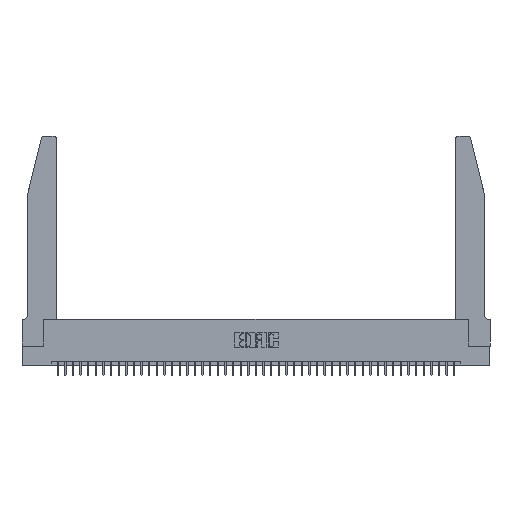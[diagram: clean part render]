
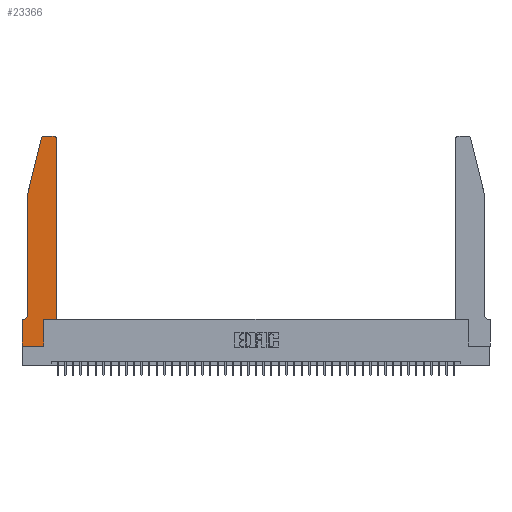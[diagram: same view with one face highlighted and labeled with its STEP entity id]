
A CAD part, top view. The second image highlights one B-rep face of the part: STEP entity #23366.
In plain terms, the highlighted planar face has unit normal (0, 0, 1).
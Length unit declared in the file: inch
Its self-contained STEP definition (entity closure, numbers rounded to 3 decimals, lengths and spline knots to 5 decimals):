
#129 = DIRECTION ( 'NONE',  ( 0., 1., 0. ) ) ;
#904 = ORIENTED_EDGE ( 'NONE', *, *, #10181, .T. ) ;
#1175 = ORIENTED_EDGE ( 'NONE', *, *, #5664, .T. ) ;
#2335 = ORIENTED_EDGE ( 'NONE', *, *, #37423, .T. ) ;
#2503 = LINE ( 'NONE', #16381, #4380 ) ;
#2833 = DIRECTION ( 'NONE',  ( 1., 0., 0. ) ) ;
#3276 = AXIS2_PLACEMENT_3D ( 'NONE', #43817, #40425, #36788 ) ;
#3529 = AXIS2_PLACEMENT_3D ( 'NONE', #12852, #26526, #24025 ) ;
#3809 = CARTESIAN_POINT ( 'NONE',  ( 0., 0.35, 0.37 ) ) ;
#4298 = VERTEX_POINT ( 'NONE', #38817 ) ;
#4380 = VECTOR ( 'NONE', #23457, 39.37008 ) ;
#5245 = LINE ( 'NONE', #39628, #39084 ) ;
#5451 = ORIENTED_EDGE ( 'NONE', *, *, #40570, .T. ) ;
#5664 = EDGE_CURVE ( 'NONE', #42920, #33251, #24505, .T. ) ;
#5913 = DIRECTION ( 'NONE',  ( 0., 1., 0. ) ) ;
#5973 = LINE ( 'NONE', #8941, #38480 ) ;
#6013 = LINE ( 'NONE', #20572, #33003 ) ;
#7016 = EDGE_CURVE ( 'NONE', #10282, #26525, #2503, .T. ) ;
#7324 = CARTESIAN_POINT ( 'NONE',  ( 0.2865, 0.35, 0.37 ) ) ;
#7619 = EDGE_CURVE ( 'NONE', #35873, #39722, #5973, .T. ) ;
#7812 = EDGE_LOOP ( 'NONE', ( #14231, #904, #12488, #36674, #24455, #23927, #14611, #23349, #5451, #9015, #1175, #2335 ) ) ;
#8283 = VECTOR ( 'NONE', #10726, 39.37008 ) ;
#8941 = CARTESIAN_POINT ( 'NONE',  ( 0.2605, 2.75, 0.37 ) ) ;
#9015 = ORIENTED_EDGE ( 'NONE', *, *, #35864, .T. ) ;
#9050 = CARTESIAN_POINT ( 'NONE',  ( 0.0755, 0.35, 0.37 ) ) ;
#9737 = CARTESIAN_POINT ( 'NONE',  ( 0.4205, 2.75, 0.37 ) ) ;
#9838 = DIRECTION ( 'NONE',  ( 0., -1., 0. ) ) ;
#10181 = EDGE_CURVE ( 'NONE', #39722, #10282, #28650, .T. ) ;
#10210 = DIRECTION ( 'NONE',  ( 1., 0., 0. ) ) ;
#10282 = VERTEX_POINT ( 'NONE', #36756 ) ;
#10448 = EDGE_CURVE ( 'NONE', #4298, #36068, #6013, .T. ) ;
#10726 = DIRECTION ( 'NONE',  ( 0., -1., 0. ) ) ;
#11253 = CIRCLE ( 'NONE', #3276, 0.03 ) ;
#11283 = CARTESIAN_POINT ( 'NONE',  ( 0.2865, 0., 0.37 ) ) ;
#12488 = ORIENTED_EDGE ( 'NONE', *, *, #7016, .T. ) ;
#12852 = CARTESIAN_POINT ( 'NONE',  ( 0.0055, 0.42, 0.37 ) ) ;
#12903 = DIRECTION ( 'NONE',  ( -1., 0., 0. ) ) ;
#14231 = ORIENTED_EDGE ( 'NONE', *, *, #7619, .T. ) ;
#14611 = ORIENTED_EDGE ( 'NONE', *, *, #40240, .T. ) ;
#15180 = CARTESIAN_POINT ( 'NONE',  ( 0.0755, 0.42, 0.37 ) ) ;
#15213 = VECTOR ( 'NONE', #129, 39.37008 ) ;
#16381 = CARTESIAN_POINT ( 'NONE',  ( 0.0755, 2., 0.37 ) ) ;
#16571 = CARTESIAN_POINT ( 'NONE',  ( 0.0055, 0.35, 0.37 ) ) ;
#16766 = VERTEX_POINT ( 'NONE', #3809 ) ;
#16777 = CARTESIAN_POINT ( 'NONE',  ( 0., 0.35, 0.37 ) ) ;
#17036 = DIRECTION ( 'NONE',  ( 0., 0., 1. ) ) ;
#20313 = LINE ( 'NONE', #41241, #44854 ) ;
#20572 = CARTESIAN_POINT ( 'NONE',  ( 0., 0., 0.37 ) ) ;
#20675 = CARTESIAN_POINT ( 'NONE',  ( 0.284, 2.72, 0.37 ) ) ;
#21361 = AXIS2_PLACEMENT_3D ( 'NONE', #20675, #17036, #10210 ) ;
#21593 = CIRCLE ( 'NONE', #3529, 0.07 ) ;
#22819 = VECTOR ( 'NONE', #26368, 39.37008 ) ;
#23219 = CARTESIAN_POINT ( 'NONE',  ( 0.4505, 0.35, 0.37 ) ) ;
#23349 = ORIENTED_EDGE ( 'NONE', *, *, #10448, .T. ) ;
#23366 = ADVANCED_FACE ( 'NONE', ( #23626 ), #34074, .T. ) ;
#23457 = DIRECTION ( 'NONE',  ( -0.239, -0.971, 0. ) ) ;
#23626 = FACE_OUTER_BOUND ( 'NONE', #7812, .T. ) ;
#23636 = LINE ( 'NONE', #37508, #22819 ) ;
#23927 = ORIENTED_EDGE ( 'NONE', *, *, #34401, .T. ) ;
#24025 = DIRECTION ( 'NONE',  ( -1., 0., 0. ) ) ;
#24455 = ORIENTED_EDGE ( 'NONE', *, *, #41676, .T. ) ;
#24505 = LINE ( 'NONE', #31543, #15213 ) ;
#26357 = AXIS2_PLACEMENT_3D ( 'NONE', #16777, #29782, #33623 ) ;
#26368 = DIRECTION ( 'NONE',  ( 1., 0., 0. ) ) ;
#26525 = VERTEX_POINT ( 'NONE', #44440 ) ;
#26526 = DIRECTION ( 'NONE',  ( 0., 0., -1. ) ) ;
#28650 = CIRCLE ( 'NONE', #21361, 0.03 ) ;
#29678 = DIRECTION ( 'NONE',  ( -1., 0., 0. ) ) ;
#29782 = DIRECTION ( 'NONE',  ( 0., 0., 1. ) ) ;
#31009 = VERTEX_POINT ( 'NONE', #16571 ) ;
#31230 = CARTESIAN_POINT ( 'NONE',  ( 0.0755, 2., 0.37 ) ) ;
#31543 = CARTESIAN_POINT ( 'NONE',  ( 0.4505, 0.35, 0.37 ) ) ;
#32774 = VERTEX_POINT ( 'NONE', #15180 ) ;
#33003 = VECTOR ( 'NONE', #2833, 39.37008 ) ;
#33251 = VERTEX_POINT ( 'NONE', #43557 ) ;
#33623 = DIRECTION ( 'NONE',  ( 1., 0., 0. ) ) ;
#34074 = PLANE ( 'NONE',  #26357 ) ;
#34401 = EDGE_CURVE ( 'NONE', #31009, #16766, #40232, .T. ) ;
#34977 = VERTEX_POINT ( 'NONE', #7324 ) ;
#35085 = EDGE_CURVE ( 'NONE', #26525, #32774, #41904, .T. ) ;
#35864 = EDGE_CURVE ( 'NONE', #34977, #42920, #23636, .T. ) ;
#35873 = VERTEX_POINT ( 'NONE', #9737 ) ;
#36068 = VERTEX_POINT ( 'NONE', #11283 ) ;
#36674 = ORIENTED_EDGE ( 'NONE', *, *, #35085, .T. ) ;
#36756 = CARTESIAN_POINT ( 'NONE',  ( 0.25487, 2.72718, 0.37 ) ) ;
#36788 = DIRECTION ( 'NONE',  ( 1., 0., 0. ) ) ;
#37423 = EDGE_CURVE ( 'NONE', #33251, #35873, #11253, .T. ) ;
#37508 = CARTESIAN_POINT ( 'NONE',  ( 0.4505, 0.35, 0.37 ) ) ;
#38480 = VECTOR ( 'NONE', #29678, 39.37008 ) ;
#38817 = CARTESIAN_POINT ( 'NONE',  ( 0., 0., 0.37 ) ) ;
#39084 = VECTOR ( 'NONE', #5913, 39.37008 ) ;
#39628 = CARTESIAN_POINT ( 'NONE',  ( 0.2865, 0.35, 0.37 ) ) ;
#39722 = VERTEX_POINT ( 'NONE', #42737 ) ;
#40232 = LINE ( 'NONE', #9050, #41712 ) ;
#40240 = EDGE_CURVE ( 'NONE', #16766, #4298, #20313, .T. ) ;
#40425 = DIRECTION ( 'NONE',  ( 0., 0., 1. ) ) ;
#40570 = EDGE_CURVE ( 'NONE', #36068, #34977, #5245, .T. ) ;
#41241 = CARTESIAN_POINT ( 'NONE',  ( 0., 0., 0.37 ) ) ;
#41676 = EDGE_CURVE ( 'NONE', #32774, #31009, #21593, .T. ) ;
#41712 = VECTOR ( 'NONE', #12903, 39.37008 ) ;
#41904 = LINE ( 'NONE', #31230, #8283 ) ;
#42737 = CARTESIAN_POINT ( 'NONE',  ( 0.284, 2.75, 0.37 ) ) ;
#42920 = VERTEX_POINT ( 'NONE', #23219 ) ;
#43557 = CARTESIAN_POINT ( 'NONE',  ( 0.4505, 2.72, 0.37 ) ) ;
#43817 = CARTESIAN_POINT ( 'NONE',  ( 0.4205, 2.72, 0.37 ) ) ;
#44440 = CARTESIAN_POINT ( 'NONE',  ( 0.0755, 2., 0.37 ) ) ;
#44854 = VECTOR ( 'NONE', #9838, 39.37008 ) ;
